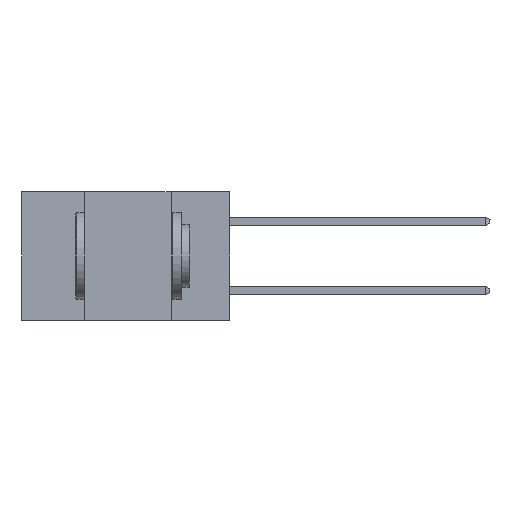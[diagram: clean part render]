
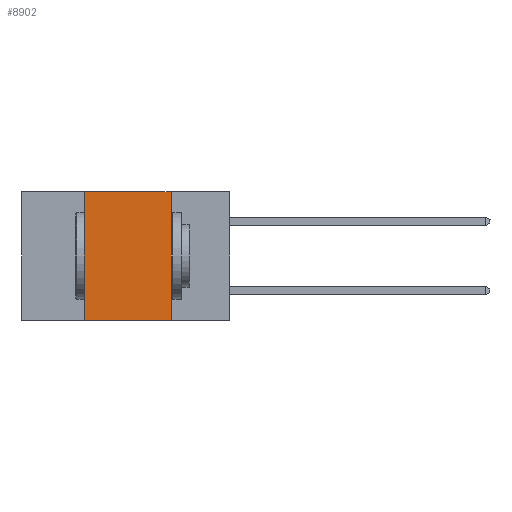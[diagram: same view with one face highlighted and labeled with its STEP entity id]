
A CAD part, left-side view. The second image highlights one B-rep face of the part: STEP entity #8902.
In plain terms, the highlighted planar face has unit normal (-1, 0, 0).
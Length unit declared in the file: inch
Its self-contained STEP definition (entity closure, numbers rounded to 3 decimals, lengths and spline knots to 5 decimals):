
#1314 = VECTOR ( 'NONE', #18964, 39.37008 ) ;
#1844 = VECTOR ( 'NONE', #13685, 39.37008 ) ;
#1935 = EDGE_CURVE ( 'NONE', #12512, #3239, #18310, .T. ) ;
#2408 = EDGE_LOOP ( 'NONE', ( #16814, #12610, #7937, #6035 ) ) ;
#2420 = VECTOR ( 'NONE', #13109, 39.37008 ) ;
#2569 = PLANE ( 'NONE',  #14963 ) ;
#2976 = CARTESIAN_POINT ( 'NONE',  ( 0., 0.17, 0. ) ) ;
#3239 = VERTEX_POINT ( 'NONE', #11581 ) ;
#5553 = DIRECTION ( 'NONE',  ( 0., 0., -1. ) ) ;
#6035 = ORIENTED_EDGE ( 'NONE', *, *, #7393, .T. ) ;
#7393 = EDGE_CURVE ( 'NONE', #12512, #14757, #13547, .T. ) ;
#7812 = CARTESIAN_POINT ( 'NONE',  ( 0., 0.6, 0. ) ) ;
#7937 = ORIENTED_EDGE ( 'NONE', *, *, #1935, .F. ) ;
#8902 = ADVANCED_FACE ( 'NONE', ( #18836 ), #2569, .F. ) ;
#9329 = CARTESIAN_POINT ( 'NONE',  ( 0., 0.42, 0. ) ) ;
#9932 = VECTOR ( 'NONE', #12283, 39.37008 ) ;
#11581 = CARTESIAN_POINT ( 'NONE',  ( 0., 0.42, 0. ) ) ;
#11648 = CARTESIAN_POINT ( 'NONE',  ( 0., 0.42, -0.37 ) ) ;
#12214 = LINE ( 'NONE', #7812, #1844 ) ;
#12283 = DIRECTION ( 'NONE',  ( 0., 0., 1. ) ) ;
#12512 = VERTEX_POINT ( 'NONE', #11648 ) ;
#12610 = ORIENTED_EDGE ( 'NONE', *, *, #14591, .F. ) ;
#12864 = DIRECTION ( 'NONE',  ( 1., 0., 0. ) ) ;
#13109 = DIRECTION ( 'NONE',  ( 0., 0., -1. ) ) ;
#13136 = CARTESIAN_POINT ( 'NONE',  ( 0., 0.6, 0. ) ) ;
#13547 = LINE ( 'NONE', #15772, #1314 ) ;
#13685 = DIRECTION ( 'NONE',  ( 0., -1., 0. ) ) ;
#14405 = LINE ( 'NONE', #14653, #2420 ) ;
#14591 = EDGE_CURVE ( 'NONE', #3239, #15410, #12214, .T. ) ;
#14653 = CARTESIAN_POINT ( 'NONE',  ( 0., 0.17, 0. ) ) ;
#14757 = VERTEX_POINT ( 'NONE', #17702 ) ;
#14963 = AXIS2_PLACEMENT_3D ( 'NONE', #13136, #12864, #5553 ) ;
#15410 = VERTEX_POINT ( 'NONE', #2976 ) ;
#15772 = CARTESIAN_POINT ( 'NONE',  ( 0., 0.6, -0.37 ) ) ;
#16289 = EDGE_CURVE ( 'NONE', #15410, #14757, #14405, .T. ) ;
#16814 = ORIENTED_EDGE ( 'NONE', *, *, #16289, .F. ) ;
#17702 = CARTESIAN_POINT ( 'NONE',  ( 0., 0.17, -0.37 ) ) ;
#18310 = LINE ( 'NONE', #9329, #9932 ) ;
#18836 = FACE_OUTER_BOUND ( 'NONE', #2408, .T. ) ;
#18964 = DIRECTION ( 'NONE',  ( 0., -1., 0. ) ) ;
